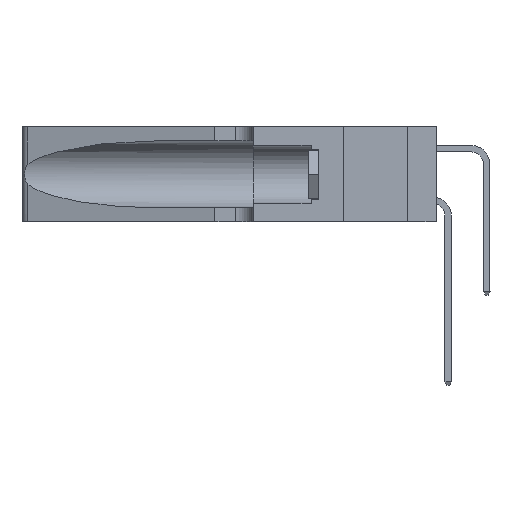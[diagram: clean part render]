
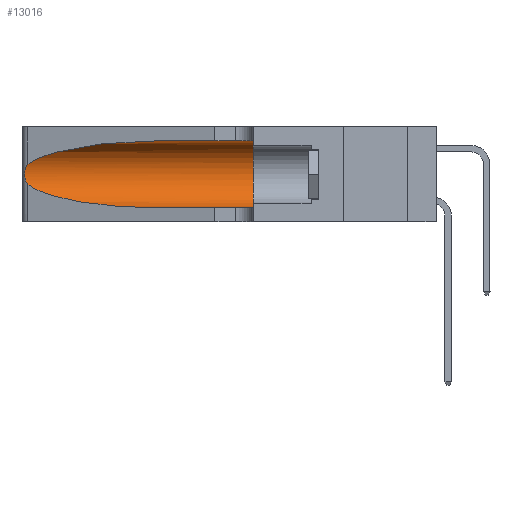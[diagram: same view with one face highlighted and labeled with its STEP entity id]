
A CAD part, left-side view. The second image highlights one B-rep face of the part: STEP entity #13016.
In plain terms, the highlighted cylindrical face has radius 3.308 mm (diameter 6.617 mm), a partial arc.
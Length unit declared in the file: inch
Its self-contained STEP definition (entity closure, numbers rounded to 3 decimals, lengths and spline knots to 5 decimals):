
#301 = EDGE_CURVE ( 'NONE', #11918, #16954, #12468, .T. ) ;
#697 = CARTESIAN_POINT ( 'NONE',  ( 0.25487, 1.22718, 0.22369 ) ) ;
#1333 = CARTESIAN_POINT ( 'NONE',  ( 0.25487, 1.22718, 0.14631 ) ) ;
#1567 = CARTESIAN_POINT ( 'NONE',  ( 0.26075, 1.23896, 0.178 ) ) ;
#1933 = CARTESIAN_POINT ( 'NONE',  ( 0.2373, 1.15595, 0.08982 ) ) ;
#3277 = CARTESIAN_POINT ( 'NONE',  ( 0.25854, 1.2359, 0.20912 ) ) ;
#3431 = CARTESIAN_POINT ( 'NONE',  ( 0.18966, 0.96281, 0.05475 ) ) ;
#4302 = ORIENTED_EDGE ( 'NONE', *, *, #7511, .T. ) ;
#4533 =( BOUNDED_CURVE ( )  B_SPLINE_CURVE ( 3, ( #18463, #18534, #15545, #18884 ),
 .UNSPECIFIED., .F., .F. ) 
 B_SPLINE_CURVE_WITH_KNOTS ( ( 4, 4 ),
 ( 1.5708, 2.84003 ),
 .UNSPECIFIED. ) 
 CURVE ( )  GEOMETRIC_REPRESENTATION_ITEM ( )  RATIONAL_B_SPLINE_CURVE ( ( 1., 0.87, 0.87, 1. ) ) 
 REPRESENTATION_ITEM ( '' )  );
#4658 = CARTESIAN_POINT ( 'NONE',  ( 0.1305, 0.35, 0.31525 ) ) ;
#4843 = CARTESIAN_POINT ( 'NONE',  ( 0.25639, 1.23184, 0.21858 ) ) ;
#4889 = ORIENTED_EDGE ( 'NONE', *, *, #9811, .F. ) ;
#5367 = CARTESIAN_POINT ( 'NONE',  ( 0.1305, 0.72297, 0.05475 ) ) ;
#5927 = FACE_OUTER_BOUND ( 'NONE', #8704, .T. ) ;
#6507 = CARTESIAN_POINT ( 'NONE',  ( 0.25555, 1.22994, 0.2215 ) ) ;
#7511 = EDGE_CURVE ( 'NONE', #11591, #11918, #9192, .T. ) ;
#7615 = AXIS2_PLACEMENT_3D ( 'NONE', #9091, #14346, #16116 ) ;
#7683 = CARTESIAN_POINT ( 'NONE',  ( 0.1305, 0.35, 0.185 ) ) ;
#7765 = ORIENTED_EDGE ( 'NONE', *, *, #301, .T. ) ;
#7991 = CARTESIAN_POINT ( 'NONE',  ( 0.1305, 0.72297, 0.31525 ) ) ;
#8176 = EDGE_CURVE ( 'NONE', #13632, #11591, #4533, .T. ) ;
#8307 = CARTESIAN_POINT ( 'NONE',  ( 0.26017, 1.23833, 0.17102 ) ) ;
#8384 = CARTESIAN_POINT ( 'NONE',  ( 0.25856, 1.23593, 0.16098 ) ) ;
#8456 = CARTESIAN_POINT ( 'NONE',  ( 0.25787, 1.23484, 0.2124 ) ) ;
#8704 = EDGE_LOOP ( 'NONE', ( #14477, #4302, #7765, #10253, #10902, #4889 ) ) ;
#9023 = VECTOR ( 'NONE', #17783, 39.37008 ) ;
#9091 = CARTESIAN_POINT ( 'NONE',  ( 0.1305, 1.61858, 0.185 ) ) ;
#9175 = CARTESIAN_POINT ( 'NONE',  ( 0.25487, 1.22718, 0.14631 ) ) ;
#9192 = B_SPLINE_CURVE_WITH_KNOTS ( 'NONE', 3,
 ( #11862, #6507, #4843, #8456, #3277, #16716, #10130, #1567, #8307, #8384, #20120, #13422, #11565, #1333 ),
 .UNSPECIFIED., .F., .F.,
 ( 4, 2, 2, 2, 2, 2, 4 ),
 ( 0., 0.00027, 0.00053, 0.00107, 0.0016, 0.00187, 0.00214 ),
 .UNSPECIFIED. ) ;
#9811 = EDGE_CURVE ( 'NONE', #13632, #17644, #18272, .T. ) ;
#10130 = CARTESIAN_POINT ( 'NONE',  ( 0.26075, 1.23896, 0.19203 ) ) ;
#10240 = LINE ( 'NONE', #20420, #21614 ) ;
#10253 = ORIENTED_EDGE ( 'NONE', *, *, #15911, .T. ) ;
#10902 = ORIENTED_EDGE ( 'NONE', *, *, #21663, .F. ) ;
#11565 = CARTESIAN_POINT ( 'NONE',  ( 0.25555, 1.22993, 0.14849 ) ) ;
#11591 = VERTEX_POINT ( 'NONE', #697 ) ;
#11862 = CARTESIAN_POINT ( 'NONE',  ( 0.25487, 1.22718, 0.22369 ) ) ;
#11918 = VERTEX_POINT ( 'NONE', #9175 ) ;
#12468 =( BOUNDED_CURVE ( )  B_SPLINE_CURVE ( 3, ( #12617, #1933, #3431, #5367 ),
 .UNSPECIFIED., .F., .F. ) 
 B_SPLINE_CURVE_WITH_KNOTS ( ( 4, 4 ),
 ( 3.44316, 4.71239 ),
 .UNSPECIFIED. ) 
 CURVE ( )  GEOMETRIC_REPRESENTATION_ITEM ( )  RATIONAL_B_SPLINE_CURVE ( ( 1., 0.87, 0.87, 1. ) ) 
 REPRESENTATION_ITEM ( '' )  );
#12617 = CARTESIAN_POINT ( 'NONE',  ( 0.25487, 1.22718, 0.14631 ) ) ;
#13016 = ADVANCED_FACE ( 'NONE', ( #5927 ), #19152, .F. ) ;
#13246 = VERTEX_POINT ( 'NONE', #13468 ) ;
#13422 = CARTESIAN_POINT ( 'NONE',  ( 0.25639, 1.23186, 0.15144 ) ) ;
#13468 = CARTESIAN_POINT ( 'NONE',  ( 0.1305, 0.35, 0.05475 ) ) ;
#13632 = VERTEX_POINT ( 'NONE', #7991 ) ;
#14346 = DIRECTION ( 'NONE',  ( 0., -1., 0. ) ) ;
#14477 = ORIENTED_EDGE ( 'NONE', *, *, #8176, .T. ) ;
#14859 = CARTESIAN_POINT ( 'NONE',  ( 0.1305, 0.72297, 0.05475 ) ) ;
#15248 = DIRECTION ( 'NONE',  ( 0., -1., 0. ) ) ;
#15545 = CARTESIAN_POINT ( 'NONE',  ( 0.2373, 1.15595, 0.28018 ) ) ;
#15911 = EDGE_CURVE ( 'NONE', #16954, #13246, #10240, .T. ) ;
#16116 = DIRECTION ( 'NONE',  ( 0., 0., -1. ) ) ;
#16332 = DIRECTION ( 'NONE',  ( 0., 1., 0. ) ) ;
#16716 = CARTESIAN_POINT ( 'NONE',  ( 0.26018, 1.23835, 0.19895 ) ) ;
#16954 = VERTEX_POINT ( 'NONE', #14859 ) ;
#17644 = VERTEX_POINT ( 'NONE', #4658 ) ;
#17783 = DIRECTION ( 'NONE',  ( 0., -1., 0. ) ) ;
#17860 = CARTESIAN_POINT ( 'NONE',  ( 0.1305, 1.61858, 0.31525 ) ) ;
#17871 = DIRECTION ( 'NONE',  ( 0., 0., 1. ) ) ;
#18272 = LINE ( 'NONE', #17860, #9023 ) ;
#18463 = CARTESIAN_POINT ( 'NONE',  ( 0.1305, 0.72297, 0.31525 ) ) ;
#18534 = CARTESIAN_POINT ( 'NONE',  ( 0.18966, 0.96281, 0.31525 ) ) ;
#18884 = CARTESIAN_POINT ( 'NONE',  ( 0.25487, 1.22718, 0.22369 ) ) ;
#19152 = CYLINDRICAL_SURFACE ( 'NONE', #7615, 0.13025 ) ;
#20120 = CARTESIAN_POINT ( 'NONE',  ( 0.25789, 1.23486, 0.15765 ) ) ;
#20234 = CIRCLE ( 'NONE', #21598, 0.13025 ) ;
#20420 = CARTESIAN_POINT ( 'NONE',  ( 0.1305, 1.61858, 0.05475 ) ) ;
#21598 = AXIS2_PLACEMENT_3D ( 'NONE', #7683, #16332, #17871 ) ;
#21614 = VECTOR ( 'NONE', #15248, 39.37008 ) ;
#21663 = EDGE_CURVE ( 'NONE', #17644, #13246, #20234, .T. ) ;
